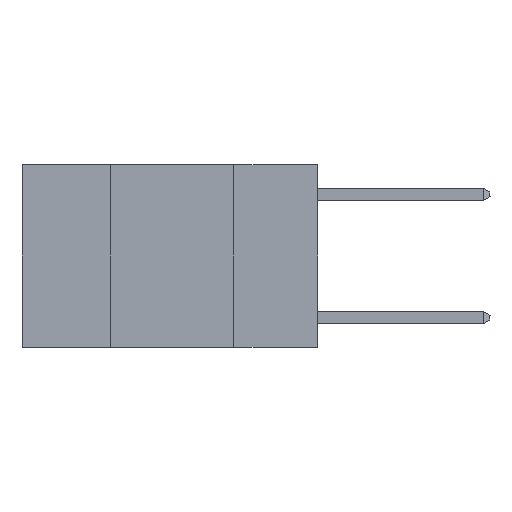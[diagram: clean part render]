
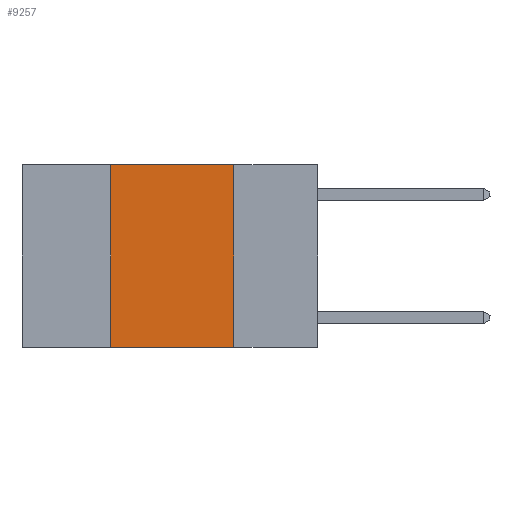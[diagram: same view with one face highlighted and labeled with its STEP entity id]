
A CAD part, left-side view. The second image highlights one B-rep face of the part: STEP entity #9257.
In plain terms, the highlighted planar face has unit normal (-1, 0, 0).
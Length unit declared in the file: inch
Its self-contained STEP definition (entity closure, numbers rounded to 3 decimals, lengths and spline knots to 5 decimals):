
#72 = VERTEX_POINT ( 'NONE', #12159 ) ;
#311 = CARTESIAN_POINT ( 'NONE',  ( 0., 0.17, -0.37 ) ) ;
#566 = ORIENTED_EDGE ( 'NONE', *, *, #27382, .F. ) ;
#723 = DIRECTION ( 'NONE',  ( 0., 0., -1. ) ) ;
#1174 = CARTESIAN_POINT ( 'NONE',  ( 0., 0.17, 0. ) ) ;
#1387 = EDGE_CURVE ( 'NONE', #16940, #17144, #24506, .T. ) ;
#1483 = VECTOR ( 'NONE', #723, 39.37008 ) ;
#3565 = ORIENTED_EDGE ( 'NONE', *, *, #10499, .F. ) ;
#5513 = DIRECTION ( 'NONE',  ( 1., 0., 0. ) ) ;
#6388 = AXIS2_PLACEMENT_3D ( 'NONE', #12663, #5513, #10677 ) ;
#6494 = DIRECTION ( 'NONE',  ( 0., -1., 0. ) ) ;
#7098 = LINE ( 'NONE', #27838, #24190 ) ;
#7786 = PLANE ( 'NONE',  #6388 ) ;
#8606 = CARTESIAN_POINT ( 'NONE',  ( 0., 0.6, -0.37 ) ) ;
#9257 = ADVANCED_FACE ( 'NONE', ( #22273 ), #7786, .F. ) ;
#10499 = EDGE_CURVE ( 'NONE', #14124, #72, #19200, .T. ) ;
#10677 = DIRECTION ( 'NONE',  ( 0., 0., -1. ) ) ;
#12088 = CARTESIAN_POINT ( 'NONE',  ( 0., 0.42, -0.37 ) ) ;
#12159 = CARTESIAN_POINT ( 'NONE',  ( 0., 0.42, 0. ) ) ;
#12663 = CARTESIAN_POINT ( 'NONE',  ( 0., 0.6, 0. ) ) ;
#14124 = VERTEX_POINT ( 'NONE', #12088 ) ;
#15694 = CARTESIAN_POINT ( 'NONE',  ( 0., 0.17, 0. ) ) ;
#16774 = CARTESIAN_POINT ( 'NONE',  ( 0., 0.42, 0. ) ) ;
#16940 = VERTEX_POINT ( 'NONE', #15694 ) ;
#17144 = VERTEX_POINT ( 'NONE', #311 ) ;
#17897 = DIRECTION ( 'NONE',  ( 0., -1., 0. ) ) ;
#19103 = EDGE_CURVE ( 'NONE', #14124, #17144, #29520, .T. ) ;
#19200 = LINE ( 'NONE', #16774, #22974 ) ;
#22273 = FACE_OUTER_BOUND ( 'NONE', #25660, .T. ) ;
#22974 = VECTOR ( 'NONE', #27960, 39.37008 ) ;
#24190 = VECTOR ( 'NONE', #6494, 39.37008 ) ;
#24506 = LINE ( 'NONE', #1174, #1483 ) ;
#25660 = EDGE_LOOP ( 'NONE', ( #29931, #566, #3565, #28999 ) ) ;
#27382 = EDGE_CURVE ( 'NONE', #72, #16940, #7098, .T. ) ;
#27588 = VECTOR ( 'NONE', #17897, 39.37008 ) ;
#27838 = CARTESIAN_POINT ( 'NONE',  ( 0., 0.6, 0. ) ) ;
#27960 = DIRECTION ( 'NONE',  ( 0., 0., 1. ) ) ;
#28999 = ORIENTED_EDGE ( 'NONE', *, *, #19103, .T. ) ;
#29520 = LINE ( 'NONE', #8606, #27588 ) ;
#29931 = ORIENTED_EDGE ( 'NONE', *, *, #1387, .F. ) ;
